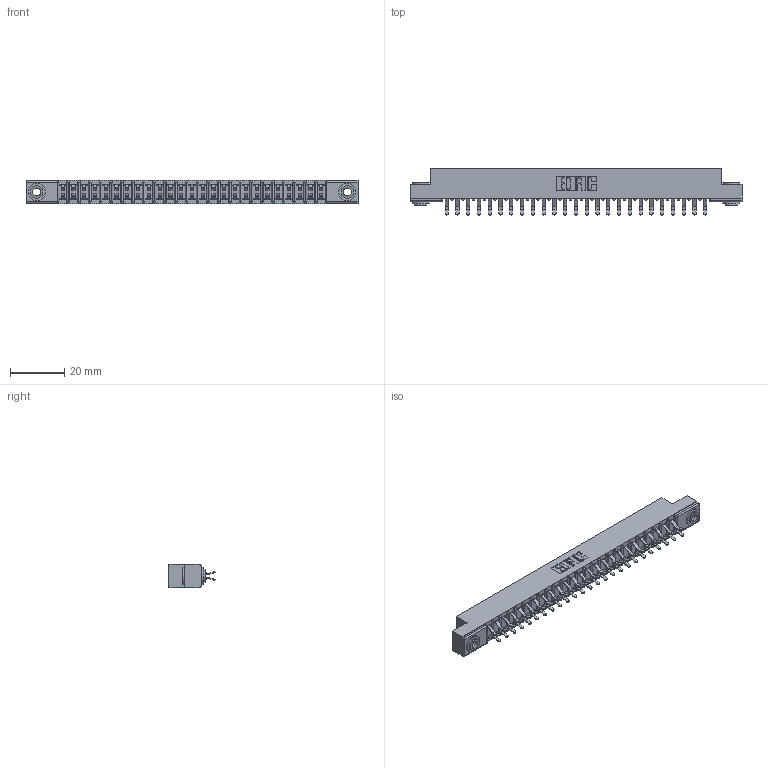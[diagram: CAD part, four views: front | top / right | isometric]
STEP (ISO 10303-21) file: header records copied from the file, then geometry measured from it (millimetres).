
FILE_DESCRIPTION (( 'STEP AP203' ), '1' );
FILE_NAME ('357-050-556-203.STEP', '2019-09-19T02:54:24', ( '' ), ( '' ), 'SwSTEP 2.0', 'SolidWorks 2016', '' );
FILE_SCHEMA (( 'CONFIG_CONTROL_DESIGN' ));
Length unit declared in the file: inch
Products named in the file (4): 357-050-556-203; 307-290-001_556; 307 Part_.156 Dia Mounting Holes; 345-250-002_345-250-002-102
Assembly tree (53 placements, depth 2):
  357-050-556-203
    307 Part_.156 Dia Mounting Holes
    307-290-001_556  x50
    345-250-002_345-250-002-102  x2
Bounding box: 122.07 x 16.97 x 8.71 mm (x, y, z)
Volume: 7976.7 mm3; surface area: 14442.6 mm2
Topology: 53 solids, 53 shells, 2696 faces, 7535 edges, 4882 vertices
Faces by surface type: plane 1744, cylinder 892, sphere 52, cone 8
Entity records: 25497 total; most frequent: CARTESIAN_POINT 4158, ORIENTED_EDGE 4110, DIRECTION 4095, EDGE_CURVE 2055, VECTOR 1561, LINE 1561, VERTEX_POINT 1330, AXIS2_PLACEMENT_3D 1267
